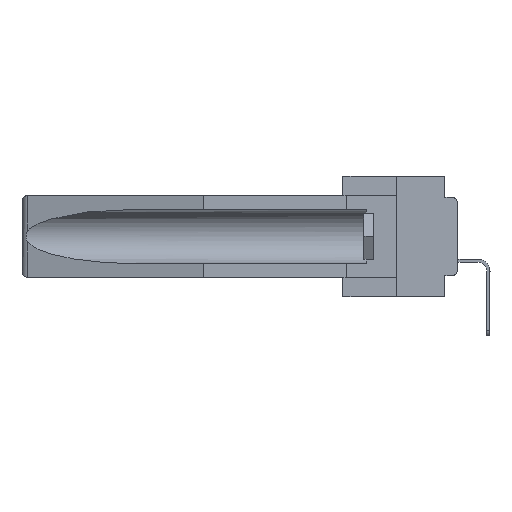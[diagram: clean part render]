
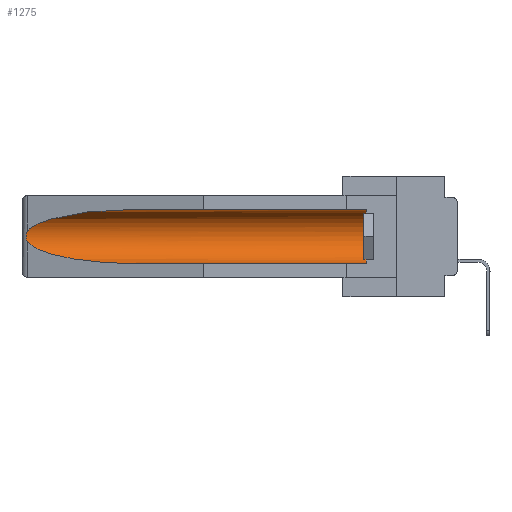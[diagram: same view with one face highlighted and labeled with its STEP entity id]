
A CAD part, left-side view. The second image highlights one B-rep face of the part: STEP entity #1275.
In plain terms, the highlighted cylindrical face has radius 2.857 mm (diameter 5.715 mm), a partial arc.
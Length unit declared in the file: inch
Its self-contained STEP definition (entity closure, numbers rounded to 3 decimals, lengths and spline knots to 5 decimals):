
#1275 = ADVANCED_FACE ( 'NONE', ( #29059 ), #23252, .F. ) ;
#2323 = B_SPLINE_CURVE_WITH_KNOTS ( 'NONE', 3,
 ( #16729, #6908, #26574, #11669, #11776, #14144, #26672, #9528, #9640, #4421 ),
 .UNSPECIFIED., .F., .F.,
 ( 4, 2, 2, 2, 4 ),
 ( 0., 0.00029, 0.00058, 0.00087, 0.00117 ),
 .UNSPECIFIED. ) ;
#2688 = ORIENTED_EDGE ( 'NONE', *, *, #3738, .T. ) ;
#2856 = CARTESIAN_POINT ( 'NONE',  ( 0.155, -0.30754, -0.1715 ) ) ;
#3016 = AXIS2_PLACEMENT_3D ( 'NONE', #29360, #9449, #7046 ) ;
#3114 = AXIS2_PLACEMENT_3D ( 'NONE', #2856, #27334, #24940 ) ;
#3738 = EDGE_CURVE ( 'NONE', #4940, #27933, #13782, .T. ) ;
#3757 = CARTESIAN_POINT ( 'NONE',  ( 0.25451, 1.48313, -0.09465 ) ) ;
#3784 = EDGE_CURVE ( 'NONE', #28107, #27933, #22490, .T. ) ;
#4421 = CARTESIAN_POINT ( 'NONE',  ( 0.26537, 1.52718, -0.19328 ) ) ;
#4940 = VERTEX_POINT ( 'NONE', #4953 ) ;
#4953 = CARTESIAN_POINT ( 'NONE',  ( 0.26537, 1.52718, -0.19328 ) ) ;
#6317 = CARTESIAN_POINT ( 'NONE',  ( 0.155, 1.07973, -0.059 ) ) ;
#6908 = CARTESIAN_POINT ( 'NONE',  ( 0.26597, 1.52961, -0.15275 ) ) ;
#7046 = DIRECTION ( 'NONE',  ( 0., 0., 1. ) ) ;
#8380 = ORIENTED_EDGE ( 'NONE', *, *, #20359, .T. ) ;
#9449 = DIRECTION ( 'NONE',  ( 0., -1., 0. ) ) ;
#9528 = CARTESIAN_POINT ( 'NONE',  ( 0.26655, 1.53094, -0.18657 ) ) ;
#9578 = EDGE_LOOP ( 'NONE', ( #30281, #11456, #2688, #11272, #8380, #26138 ) ) ;
#9640 = CARTESIAN_POINT ( 'NONE',  ( 0.26597, 1.5296, -0.19026 ) ) ;
#10192 = VECTOR ( 'NONE', #10214, 39.37008 ) ;
#10214 = DIRECTION ( 'NONE',  ( 0., 1., 0. ) ) ;
#11272 = ORIENTED_EDGE ( 'NONE', *, *, #3784, .F. ) ;
#11456 = ORIENTED_EDGE ( 'NONE', *, *, #13402, .T. ) ;
#11669 = CARTESIAN_POINT ( 'NONE',  ( 0.2673, 1.5327, -0.16383 ) ) ;
#11776 = CARTESIAN_POINT ( 'NONE',  ( 0.2675, 1.53308, -0.16763 ) ) ;
#12313 = CARTESIAN_POINT ( 'NONE',  ( 0.155, 0.126, -0.059 ) ) ;
#12579 = CARTESIAN_POINT ( 'NONE',  ( 0.155, -0.30754, -0.284 ) ) ;
#12966 = LINE ( 'NONE', #17605, #29165 ) ;
#13402 = EDGE_CURVE ( 'NONE', #21076, #4940, #2323, .T. ) ;
#13483 = VERTEX_POINT ( 'NONE', #12313 ) ;
#13782 =( BOUNDED_CURVE ( )  B_SPLINE_CURVE ( 3, ( #25079, #30031, #19779, #24972 ),
 .UNSPECIFIED., .F., .F. ) 
 B_SPLINE_CURVE_WITH_KNOTS ( ( 4, 4 ),
 ( 0.1948, 1.5708 ),
 .UNSPECIFIED. ) 
 CURVE ( )  GEOMETRIC_REPRESENTATION_ITEM ( )  RATIONAL_B_SPLINE_CURVE ( ( 1., 0.848, 0.848, 1. ) ) 
 REPRESENTATION_ITEM ( '' )  );
#13925 = VERTEX_POINT ( 'NONE', #16374 ) ;
#14144 = CARTESIAN_POINT ( 'NONE',  ( 0.2675, 1.53308, -0.17534 ) ) ;
#15345 = CARTESIAN_POINT ( 'NONE',  ( 0.26537, 1.52718, -0.14972 ) ) ;
#15566 = EDGE_CURVE ( 'NONE', #13483, #13925, #12966, .T. ) ;
#16374 = CARTESIAN_POINT ( 'NONE',  ( 0.155, 1.07973, -0.059 ) ) ;
#16729 = CARTESIAN_POINT ( 'NONE',  ( 0.26537, 1.52718, -0.14972 ) ) ;
#17399 = DIRECTION ( 'NONE',  ( 0., 1., 0. ) ) ;
#17605 = CARTESIAN_POINT ( 'NONE',  ( 0.155, -0.30754, -0.059 ) ) ;
#18134 = CARTESIAN_POINT ( 'NONE',  ( 0.155, 0.126, -0.284 ) ) ;
#18912 =( BOUNDED_CURVE ( )  B_SPLINE_CURVE ( 3, ( #6317, #26384, #3757, #28439 ),
 .UNSPECIFIED., .F., .F. ) 
 B_SPLINE_CURVE_WITH_KNOTS ( ( 4, 4 ),
 ( 4.71239, 6.08839 ),
 .UNSPECIFIED. ) 
 CURVE ( )  GEOMETRIC_REPRESENTATION_ITEM ( )  RATIONAL_B_SPLINE_CURVE ( ( 1., 0.848, 0.848, 1. ) ) 
 REPRESENTATION_ITEM ( '' )  );
#19779 = CARTESIAN_POINT ( 'NONE',  ( 0.21114, 1.30732, -0.284 ) ) ;
#20001 = CARTESIAN_POINT ( 'NONE',  ( 0.155, 1.07973, -0.284 ) ) ;
#20359 = EDGE_CURVE ( 'NONE', #28107, #13483, #29233, .T. ) ;
#21076 = VERTEX_POINT ( 'NONE', #15345 ) ;
#22490 = LINE ( 'NONE', #12579, #10192 ) ;
#23252 = CYLINDRICAL_SURFACE ( 'NONE', #3114, 0.1125 ) ;
#24940 = DIRECTION ( 'NONE',  ( 0., 0., 1. ) ) ;
#24972 = CARTESIAN_POINT ( 'NONE',  ( 0.155, 1.07973, -0.284 ) ) ;
#25079 = CARTESIAN_POINT ( 'NONE',  ( 0.26537, 1.52718, -0.19328 ) ) ;
#26138 = ORIENTED_EDGE ( 'NONE', *, *, #15566, .T. ) ;
#26384 = CARTESIAN_POINT ( 'NONE',  ( 0.21114, 1.30732, -0.059 ) ) ;
#26574 = CARTESIAN_POINT ( 'NONE',  ( 0.26654, 1.53092, -0.15636 ) ) ;
#26672 = CARTESIAN_POINT ( 'NONE',  ( 0.2673, 1.53269, -0.17917 ) ) ;
#27334 = DIRECTION ( 'NONE',  ( 0., 1., 0. ) ) ;
#27933 = VERTEX_POINT ( 'NONE', #20001 ) ;
#28107 = VERTEX_POINT ( 'NONE', #18134 ) ;
#28439 = CARTESIAN_POINT ( 'NONE',  ( 0.26537, 1.52718, -0.14972 ) ) ;
#29059 = FACE_OUTER_BOUND ( 'NONE', #9578, .T. ) ;
#29165 = VECTOR ( 'NONE', #17399, 39.37008 ) ;
#29233 = CIRCLE ( 'NONE', #3016, 0.1125 ) ;
#29360 = CARTESIAN_POINT ( 'NONE',  ( 0.155, 0.126, -0.1715 ) ) ;
#29637 = EDGE_CURVE ( 'NONE', #13925, #21076, #18912, .T. ) ;
#30031 = CARTESIAN_POINT ( 'NONE',  ( 0.25451, 1.48313, -0.24835 ) ) ;
#30281 = ORIENTED_EDGE ( 'NONE', *, *, #29637, .T. ) ;
